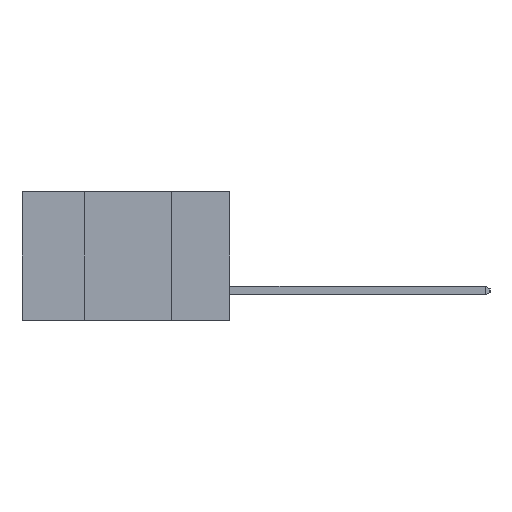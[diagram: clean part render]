
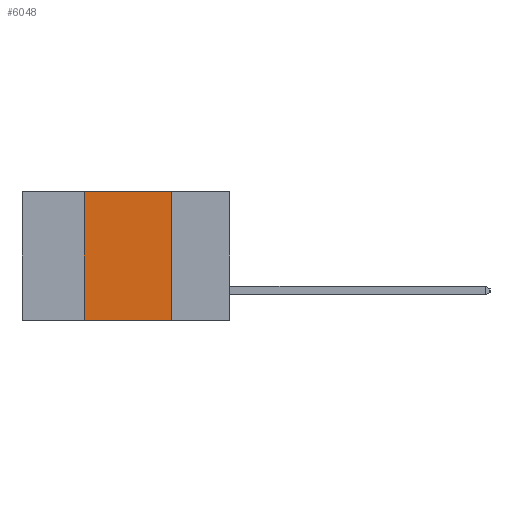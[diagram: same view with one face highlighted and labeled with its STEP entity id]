
A CAD part, left-side view. The second image highlights one B-rep face of the part: STEP entity #6048.
In plain terms, the highlighted planar face has unit normal (-1, 0, 0).
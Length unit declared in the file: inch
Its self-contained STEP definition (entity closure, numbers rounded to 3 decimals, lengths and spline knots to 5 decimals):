
#566 = VECTOR ( 'NONE', #19743, 39.37008 ) ;
#913 = EDGE_CURVE ( 'NONE', #9462, #11409, #5882, .T. ) ;
#1048 = CARTESIAN_POINT ( 'NONE',  ( 0., 0.42, 0. ) ) ;
#1274 = DIRECTION ( 'NONE',  ( 0., 0., -1. ) ) ;
#1301 = ORIENTED_EDGE ( 'NONE', *, *, #18424, .F. ) ;
#1305 = DIRECTION ( 'NONE',  ( 1., 0., 0. ) ) ;
#1542 = CARTESIAN_POINT ( 'NONE',  ( 0., 0.6, 0. ) ) ;
#1682 = PLANE ( 'NONE',  #11885 ) ;
#3547 = VECTOR ( 'NONE', #4550, 39.37008 ) ;
#4308 = CARTESIAN_POINT ( 'NONE',  ( 0., 0.42, -0.37 ) ) ;
#4550 = DIRECTION ( 'NONE',  ( 0., 0., 1. ) ) ;
#5279 = EDGE_CURVE ( 'NONE', #20239, #14994, #23755, .T. ) ;
#5314 = VECTOR ( 'NONE', #11930, 39.37008 ) ;
#5598 = ORIENTED_EDGE ( 'NONE', *, *, #913, .F. ) ;
#5882 = LINE ( 'NONE', #11317, #5314 ) ;
#6048 = ADVANCED_FACE ( 'NONE', ( #20045 ), #1682, .F. ) ;
#6721 = ORIENTED_EDGE ( 'NONE', *, *, #22074, .T. ) ;
#7183 = CARTESIAN_POINT ( 'NONE',  ( 0., 0.42, -0.37 ) ) ;
#8494 = CARTESIAN_POINT ( 'NONE',  ( 0., 0.6, -0.37 ) ) ;
#9357 = EDGE_LOOP ( 'NONE', ( #5598, #1301, #11116, #6721 ) ) ;
#9462 = VERTEX_POINT ( 'NONE', #17502 ) ;
#10361 = LINE ( 'NONE', #8494, #566 ) ;
#10377 = VECTOR ( 'NONE', #14981, 39.37008 ) ;
#11056 = CARTESIAN_POINT ( 'NONE',  ( 0., 0.17, -0.37 ) ) ;
#11116 = ORIENTED_EDGE ( 'NONE', *, *, #5279, .F. ) ;
#11317 = CARTESIAN_POINT ( 'NONE',  ( 0., 0.17, -0.37 ) ) ;
#11409 = VERTEX_POINT ( 'NONE', #11056 ) ;
#11885 = AXIS2_PLACEMENT_3D ( 'NONE', #1542, #1305, #1274 ) ;
#11930 = DIRECTION ( 'NONE',  ( 0., 0., -1. ) ) ;
#13103 = CARTESIAN_POINT ( 'NONE',  ( 0., 0.6, 0. ) ) ;
#14981 = DIRECTION ( 'NONE',  ( 0., -1., 0. ) ) ;
#14994 = VERTEX_POINT ( 'NONE', #1048 ) ;
#16584 = LINE ( 'NONE', #13103, #10377 ) ;
#17502 = CARTESIAN_POINT ( 'NONE',  ( 0., 0.17, 0. ) ) ;
#18424 = EDGE_CURVE ( 'NONE', #14994, #9462, #16584, .T. ) ;
#19743 = DIRECTION ( 'NONE',  ( 0., -1., 0. ) ) ;
#20045 = FACE_OUTER_BOUND ( 'NONE', #9357, .T. ) ;
#20239 = VERTEX_POINT ( 'NONE', #7183 ) ;
#22074 = EDGE_CURVE ( 'NONE', #20239, #11409, #10361, .T. ) ;
#23755 = LINE ( 'NONE', #4308, #3547 ) ;
